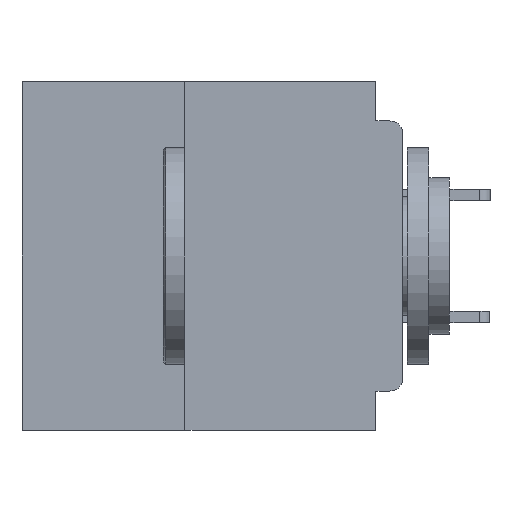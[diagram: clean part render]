
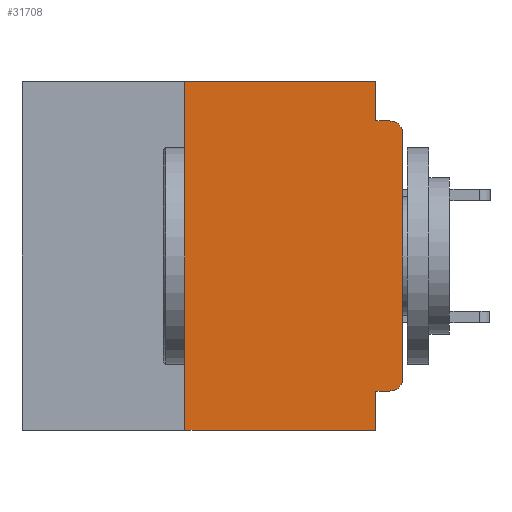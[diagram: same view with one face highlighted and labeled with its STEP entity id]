
A CAD part, left-side view. The second image highlights one B-rep face of the part: STEP entity #31708.
In plain terms, the highlighted planar face has unit normal (-1, 0, 0).
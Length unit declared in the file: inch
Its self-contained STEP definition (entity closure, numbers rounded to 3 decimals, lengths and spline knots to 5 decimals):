
#158 = LINE ( 'NONE', #29344, #50927 ) ;
#2054 = ORIENTED_EDGE ( 'NONE', *, *, #26474, .T. ) ;
#5541 = LINE ( 'NONE', #27550, #35115 ) ;
#5827 = DIRECTION ( 'NONE',  ( 0., -1., 0. ) ) ;
#5844 = EDGE_CURVE ( 'NONE', #47024, #49858, #26924, .T. ) ;
#7254 = LINE ( 'NONE', #43925, #48557 ) ;
#7587 = LINE ( 'NONE', #37817, #27728 ) ;
#7983 = CARTESIAN_POINT ( 'NONE',  ( 0., 0.015, -0.045 ) ) ;
#8013 = EDGE_CURVE ( 'NONE', #31662, #30906, #7254, .T. ) ;
#8512 = EDGE_CURVE ( 'NONE', #18371, #13252, #34111, .T. ) ;
#9123 = CARTESIAN_POINT ( 'NONE',  ( 0., 0.25, -0.4 ) ) ;
#10423 = EDGE_CURVE ( 'NONE', #17043, #10871, #18214, .T. ) ;
#10871 = VERTEX_POINT ( 'NONE', #17732 ) ;
#11872 = CARTESIAN_POINT ( 'NONE',  ( 0., 0., 0. ) ) ;
#12680 = FACE_OUTER_BOUND ( 'NONE', #30138, .T. ) ;
#13252 = VERTEX_POINT ( 'NONE', #7983 ) ;
#13399 = PLANE ( 'NONE',  #29059 ) ;
#15448 = ORIENTED_EDGE ( 'NONE', *, *, #5844, .F. ) ;
#16260 = VECTOR ( 'NONE', #21228, 39.37008 ) ;
#16589 = DIRECTION ( 'NONE',  ( -1., 0., 0. ) ) ;
#17043 = VERTEX_POINT ( 'NONE', #18602 ) ;
#17557 = EDGE_CURVE ( 'NONE', #30698, #18371, #7587, .T. ) ;
#17732 = CARTESIAN_POINT ( 'NONE',  ( 0., 0., -0.06 ) ) ;
#18214 = LINE ( 'NONE', #11872, #39519 ) ;
#18371 = VERTEX_POINT ( 'NONE', #51297 ) ;
#18500 = CARTESIAN_POINT ( 'NONE',  ( 0., 0.25, 0. ) ) ;
#18602 = CARTESIAN_POINT ( 'NONE',  ( 0., 0., -0.34 ) ) ;
#19264 = DIRECTION ( 'NONE',  ( -1., 0., 0. ) ) ;
#21228 = DIRECTION ( 'NONE',  ( 0., 0., -1. ) ) ;
#21468 = CARTESIAN_POINT ( 'NONE',  ( 0., 0.437, 0. ) ) ;
#22848 = AXIS2_PLACEMENT_3D ( 'NONE', #40530, #16589, #44526 ) ;
#24735 = AXIS2_PLACEMENT_3D ( 'NONE', #43196, #19264, #47151 ) ;
#25487 = DIRECTION ( 'NONE',  ( 0., 0., -1. ) ) ;
#26474 = EDGE_CURVE ( 'NONE', #33236, #17043, #50029, .T. ) ;
#26924 = LINE ( 'NONE', #41128, #16260 ) ;
#26989 = ORIENTED_EDGE ( 'NONE', *, *, #8013, .F. ) ;
#27165 = ORIENTED_EDGE ( 'NONE', *, *, #8512, .F. ) ;
#27550 = CARTESIAN_POINT ( 'NONE',  ( 0., 0.437, 0. ) ) ;
#27728 = VECTOR ( 'NONE', #41789, 39.37008 ) ;
#29059 = AXIS2_PLACEMENT_3D ( 'NONE', #21468, #49352, #25487 ) ;
#29344 = CARTESIAN_POINT ( 'NONE',  ( 0., 0., -0.355 ) ) ;
#30138 = EDGE_LOOP ( 'NONE', ( #34273, #50374, #27165, #49891, #30382, #26989, #51305, #15448, #34002, #2054 ) ) ;
#30382 = ORIENTED_EDGE ( 'NONE', *, *, #41699, .F. ) ;
#30698 = VERTEX_POINT ( 'NONE', #37271 ) ;
#30906 = VERTEX_POINT ( 'NONE', #18500 ) ;
#31140 = CARTESIAN_POINT ( 'NONE',  ( 0., 0.015, -0.355 ) ) ;
#31662 = VERTEX_POINT ( 'NONE', #9123 ) ;
#31708 = ADVANCED_FACE ( 'NONE', ( #12680 ), #13399, .F. ) ;
#32114 = DIRECTION ( 'NONE',  ( 0., 0., 1. ) ) ;
#33039 = EDGE_CURVE ( 'NONE', #31662, #49858, #45351, .T. ) ;
#33236 = VERTEX_POINT ( 'NONE', #31140 ) ;
#33621 = EDGE_CURVE ( 'NONE', #33236, #47024, #158, .T. ) ;
#34002 = ORIENTED_EDGE ( 'NONE', *, *, #33621, .F. ) ;
#34111 = LINE ( 'NONE', #34864, #44653 ) ;
#34273 = ORIENTED_EDGE ( 'NONE', *, *, #10423, .T. ) ;
#34833 = VECTOR ( 'NONE', #5827, 39.37008 ) ;
#34864 = CARTESIAN_POINT ( 'NONE',  ( 0., 0., -0.045 ) ) ;
#35115 = VECTOR ( 'NONE', #47384, 39.37008 ) ;
#37271 = CARTESIAN_POINT ( 'NONE',  ( 0., 0.031, 0. ) ) ;
#37817 = CARTESIAN_POINT ( 'NONE',  ( 0., 0.031, 0. ) ) ;
#38399 = CARTESIAN_POINT ( 'NONE',  ( 0., 0.031, -0.4 ) ) ;
#39050 = DIRECTION ( 'NONE',  ( 0., -1., 0. ) ) ;
#39369 = CIRCLE ( 'NONE', #24735, 0.015 ) ;
#39519 = VECTOR ( 'NONE', #39892, 39.37008 ) ;
#39892 = DIRECTION ( 'NONE',  ( 0., 0., 1. ) ) ;
#40530 = CARTESIAN_POINT ( 'NONE',  ( 0., 0.015, -0.34 ) ) ;
#41128 = CARTESIAN_POINT ( 'NONE',  ( 0., 0.031, -0.4 ) ) ;
#41699 = EDGE_CURVE ( 'NONE', #30906, #30698, #5541, .T. ) ;
#41789 = DIRECTION ( 'NONE',  ( 0., 0., -1. ) ) ;
#43196 = CARTESIAN_POINT ( 'NONE',  ( 0., 0.015, -0.06 ) ) ;
#43925 = CARTESIAN_POINT ( 'NONE',  ( 0., 0.25, -0.4 ) ) ;
#44526 = DIRECTION ( 'NONE',  ( 0., 0., -1. ) ) ;
#44653 = VECTOR ( 'NONE', #39050, 39.37008 ) ;
#45330 = DIRECTION ( 'NONE',  ( 0., 1., 0. ) ) ;
#45351 = LINE ( 'NONE', #45742, #34833 ) ;
#45742 = CARTESIAN_POINT ( 'NONE',  ( 0., 0.437, -0.4 ) ) ;
#47024 = VERTEX_POINT ( 'NONE', #51913 ) ;
#47151 = DIRECTION ( 'NONE',  ( 0., 0., -1. ) ) ;
#47384 = DIRECTION ( 'NONE',  ( 0., -1., 0. ) ) ;
#48557 = VECTOR ( 'NONE', #32114, 39.37008 ) ;
#49352 = DIRECTION ( 'NONE',  ( 1., 0., 0. ) ) ;
#49858 = VERTEX_POINT ( 'NONE', #38399 ) ;
#49891 = ORIENTED_EDGE ( 'NONE', *, *, #17557, .F. ) ;
#50029 = CIRCLE ( 'NONE', #22848, 0.015 ) ;
#50374 = ORIENTED_EDGE ( 'NONE', *, *, #50522, .T. ) ;
#50522 = EDGE_CURVE ( 'NONE', #10871, #13252, #39369, .T. ) ;
#50927 = VECTOR ( 'NONE', #45330, 39.37008 ) ;
#51297 = CARTESIAN_POINT ( 'NONE',  ( 0., 0.031, -0.045 ) ) ;
#51305 = ORIENTED_EDGE ( 'NONE', *, *, #33039, .T. ) ;
#51913 = CARTESIAN_POINT ( 'NONE',  ( 0., 0.031, -0.355 ) ) ;
